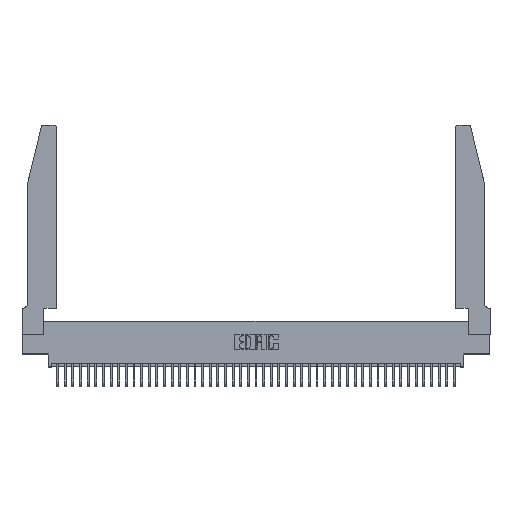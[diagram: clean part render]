
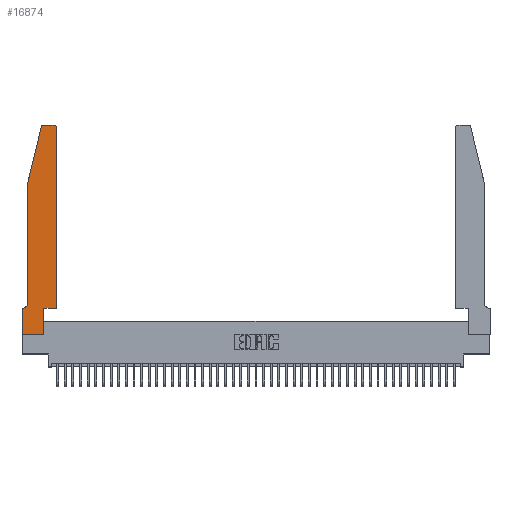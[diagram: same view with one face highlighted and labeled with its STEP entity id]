
A CAD part, top view. The second image highlights one B-rep face of the part: STEP entity #16874.
In plain terms, the highlighted planar face has unit normal (0, 0, 1).
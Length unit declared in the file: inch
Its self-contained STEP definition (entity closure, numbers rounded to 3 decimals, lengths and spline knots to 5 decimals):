
#434 = VERTEX_POINT ( 'NONE', #16311 ) ;
#1307 = VECTOR ( 'NONE', #32192, 39.37008 ) ;
#1829 = ORIENTED_EDGE ( 'NONE', *, *, #6001, .T. ) ;
#2932 = EDGE_CURVE ( 'NONE', #12791, #32086, #41292, .T. ) ;
#3034 = VECTOR ( 'NONE', #37509, 39.37008 ) ;
#3084 = LINE ( 'NONE', #12891, #35245 ) ;
#3908 = EDGE_LOOP ( 'NONE', ( #32174, #26560, #32962, #1829, #38478, #33027, #35640, #5579, #10955, #26789, #19081, #26574 ) ) ;
#4021 = AXIS2_PLACEMENT_3D ( 'NONE', #8315, #33835, #33519 ) ;
#4178 = EDGE_CURVE ( 'NONE', #32665, #434, #20675, .T. ) ;
#5160 = DIRECTION ( 'NONE',  ( 0., -1., 0. ) ) ;
#5169 = DIRECTION ( 'NONE',  ( -0.239, -0.971, 0. ) ) ;
#5435 = AXIS2_PLACEMENT_3D ( 'NONE', #9999, #41835, #16638 ) ;
#5579 = ORIENTED_EDGE ( 'NONE', *, *, #19296, .T. ) ;
#5599 = CARTESIAN_POINT ( 'NONE',  ( 0.2865, 0., 0.37 ) ) ;
#5619 = DIRECTION ( 'NONE',  ( 1., 0., 0. ) ) ;
#6001 = EDGE_CURVE ( 'NONE', #24322, #32665, #14854, .T. ) ;
#7354 = DIRECTION ( 'NONE',  ( -1., 0., 0. ) ) ;
#7659 = LINE ( 'NONE', #37680, #31927 ) ;
#8315 = CARTESIAN_POINT ( 'NONE',  ( 0.4205, 2.72, 0.37 ) ) ;
#8339 = CARTESIAN_POINT ( 'NONE',  ( 0.4505, 2.72, 0.37 ) ) ;
#8525 = CIRCLE ( 'NONE', #4021, 0.03 ) ;
#9908 = VERTEX_POINT ( 'NONE', #34162 ) ;
#9999 = CARTESIAN_POINT ( 'NONE',  ( 0., 0.35, 0.37 ) ) ;
#10941 = VECTOR ( 'NONE', #7354, 39.37008 ) ;
#10955 = ORIENTED_EDGE ( 'NONE', *, *, #29598, .T. ) ;
#12791 = VERTEX_POINT ( 'NONE', #26176 ) ;
#12865 = DIRECTION ( 'NONE',  ( 0., 0., 1. ) ) ;
#12891 = CARTESIAN_POINT ( 'NONE',  ( 0., 0., 0.37 ) ) ;
#13256 = CARTESIAN_POINT ( 'NONE',  ( 0.284, 2.75, 0.37 ) ) ;
#13373 = VECTOR ( 'NONE', #36397, 39.37008 ) ;
#13480 = CARTESIAN_POINT ( 'NONE',  ( 0.0055, 0.42, 0.37 ) ) ;
#14328 = AXIS2_PLACEMENT_3D ( 'NONE', #13480, #27211, #41833 ) ;
#14854 = LINE ( 'NONE', #38188, #3034 ) ;
#14997 = VERTEX_POINT ( 'NONE', #8339 ) ;
#15458 = CIRCLE ( 'NONE', #17109, 0.03 ) ;
#16311 = CARTESIAN_POINT ( 'NONE',  ( 0.0055, 0.35, 0.37 ) ) ;
#16418 = FACE_OUTER_BOUND ( 'NONE', #3908, .T. ) ;
#16638 = DIRECTION ( 'NONE',  ( 1., 0., 0. ) ) ;
#16763 = LINE ( 'NONE', #39733, #13373 ) ;
#16874 = ADVANCED_FACE ( 'NONE', ( #16418 ), #46071, .T. ) ;
#17109 = AXIS2_PLACEMENT_3D ( 'NONE', #31179, #12865, #5619 ) ;
#17684 = CARTESIAN_POINT ( 'NONE',  ( 0.0755, 0.35, 0.37 ) ) ;
#17726 = CARTESIAN_POINT ( 'NONE',  ( 0.0755, 0.42, 0.37 ) ) ;
#18498 = VERTEX_POINT ( 'NONE', #34916 ) ;
#18530 = CARTESIAN_POINT ( 'NONE',  ( 0.0755, 2., 0.37 ) ) ;
#19059 = VECTOR ( 'NONE', #44752, 39.37008 ) ;
#19081 = ORIENTED_EDGE ( 'NONE', *, *, #43816, .T. ) ;
#19296 = EDGE_CURVE ( 'NONE', #9908, #22729, #7659, .T. ) ;
#19699 = LINE ( 'NONE', #17684, #42256 ) ;
#20524 = EDGE_CURVE ( 'NONE', #31024, #44082, #37416, .T. ) ;
#20675 = CIRCLE ( 'NONE', #14328, 0.07 ) ;
#21120 = CARTESIAN_POINT ( 'NONE',  ( 0.4505, 0.35, 0.37 ) ) ;
#21291 = CARTESIAN_POINT ( 'NONE',  ( 0.25487, 2.72718, 0.37 ) ) ;
#21983 = EDGE_CURVE ( 'NONE', #14997, #31024, #8525, .T. ) ;
#22099 = CARTESIAN_POINT ( 'NONE',  ( 0.4205, 2.75, 0.37 ) ) ;
#22729 = VERTEX_POINT ( 'NONE', #5599 ) ;
#24215 = VECTOR ( 'NONE', #5169, 39.37008 ) ;
#24322 = VERTEX_POINT ( 'NONE', #18530 ) ;
#24594 = EDGE_CURVE ( 'NONE', #44082, #36066, #15458, .T. ) ;
#25081 = DIRECTION ( 'NONE',  ( -1., 0., 0. ) ) ;
#25274 = CARTESIAN_POINT ( 'NONE',  ( 0.4505, 0.35, 0.37 ) ) ;
#25875 = LINE ( 'NONE', #37497, #19059 ) ;
#26176 = CARTESIAN_POINT ( 'NONE',  ( 0.2865, 0.35, 0.37 ) ) ;
#26560 = ORIENTED_EDGE ( 'NONE', *, *, #24594, .T. ) ;
#26574 = ORIENTED_EDGE ( 'NONE', *, *, #21983, .T. ) ;
#26789 = ORIENTED_EDGE ( 'NONE', *, *, #2932, .T. ) ;
#27211 = DIRECTION ( 'NONE',  ( 0., 0., -1. ) ) ;
#28332 = EDGE_CURVE ( 'NONE', #434, #18498, #19699, .T. ) ;
#28650 = EDGE_CURVE ( 'NONE', #36066, #24322, #32635, .T. ) ;
#29598 = EDGE_CURVE ( 'NONE', #22729, #12791, #16763, .T. ) ;
#31024 = VERTEX_POINT ( 'NONE', #22099 ) ;
#31179 = CARTESIAN_POINT ( 'NONE',  ( 0.284, 2.72, 0.37 ) ) ;
#31927 = VECTOR ( 'NONE', #41145, 39.37008 ) ;
#32086 = VERTEX_POINT ( 'NONE', #21120 ) ;
#32174 = ORIENTED_EDGE ( 'NONE', *, *, #20524, .T. ) ;
#32192 = DIRECTION ( 'NONE',  ( 1., 0., 0. ) ) ;
#32635 = LINE ( 'NONE', #41084, #24215 ) ;
#32665 = VERTEX_POINT ( 'NONE', #17726 ) ;
#32962 = ORIENTED_EDGE ( 'NONE', *, *, #28650, .T. ) ;
#33027 = ORIENTED_EDGE ( 'NONE', *, *, #28332, .T. ) ;
#33519 = DIRECTION ( 'NONE',  ( 1., 0., 0. ) ) ;
#33835 = DIRECTION ( 'NONE',  ( 0., 0., 1. ) ) ;
#34162 = CARTESIAN_POINT ( 'NONE',  ( 0., 0., 0.37 ) ) ;
#34916 = CARTESIAN_POINT ( 'NONE',  ( 0., 0.35, 0.37 ) ) ;
#35245 = VECTOR ( 'NONE', #5160, 39.37008 ) ;
#35640 = ORIENTED_EDGE ( 'NONE', *, *, #45827, .T. ) ;
#36066 = VERTEX_POINT ( 'NONE', #21291 ) ;
#36397 = DIRECTION ( 'NONE',  ( 0., 1., 0. ) ) ;
#37416 = LINE ( 'NONE', #43435, #10941 ) ;
#37497 = CARTESIAN_POINT ( 'NONE',  ( 0.4505, 0.35, 0.37 ) ) ;
#37509 = DIRECTION ( 'NONE',  ( 0., -1., 0. ) ) ;
#37680 = CARTESIAN_POINT ( 'NONE',  ( 0., 0., 0.37 ) ) ;
#38188 = CARTESIAN_POINT ( 'NONE',  ( 0.0755, 2., 0.37 ) ) ;
#38478 = ORIENTED_EDGE ( 'NONE', *, *, #4178, .T. ) ;
#39733 = CARTESIAN_POINT ( 'NONE',  ( 0.2865, 0.35, 0.37 ) ) ;
#41084 = CARTESIAN_POINT ( 'NONE',  ( 0.0755, 2., 0.37 ) ) ;
#41145 = DIRECTION ( 'NONE',  ( 1., 0., 0. ) ) ;
#41292 = LINE ( 'NONE', #25274, #1307 ) ;
#41833 = DIRECTION ( 'NONE',  ( -1., 0., 0. ) ) ;
#41835 = DIRECTION ( 'NONE',  ( 0., 0., 1. ) ) ;
#42256 = VECTOR ( 'NONE', #25081, 39.37008 ) ;
#43435 = CARTESIAN_POINT ( 'NONE',  ( 0.2605, 2.75, 0.37 ) ) ;
#43816 = EDGE_CURVE ( 'NONE', #32086, #14997, #25875, .T. ) ;
#44082 = VERTEX_POINT ( 'NONE', #13256 ) ;
#44752 = DIRECTION ( 'NONE',  ( 0., 1., 0. ) ) ;
#45827 = EDGE_CURVE ( 'NONE', #18498, #9908, #3084, .T. ) ;
#46071 = PLANE ( 'NONE',  #5435 ) ;
